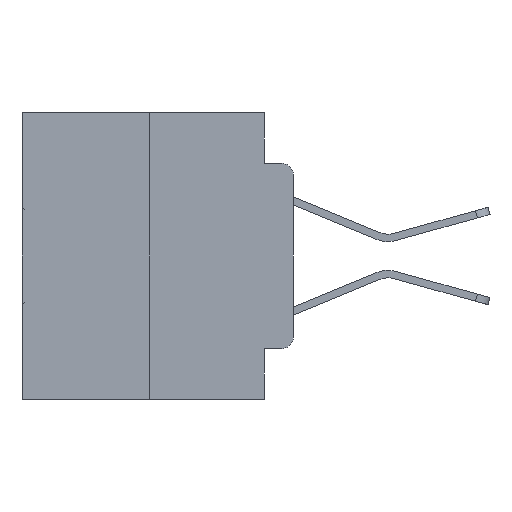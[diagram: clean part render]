
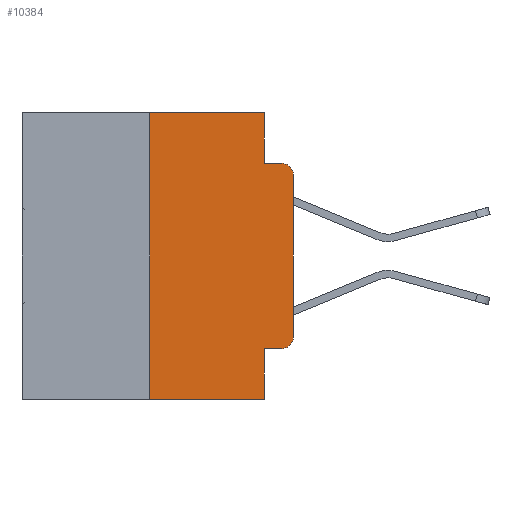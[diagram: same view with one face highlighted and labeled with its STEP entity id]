
A CAD part, left-side view. The second image highlights one B-rep face of the part: STEP entity #10384.
In plain terms, the highlighted planar face has unit normal (-1, 0, 0).
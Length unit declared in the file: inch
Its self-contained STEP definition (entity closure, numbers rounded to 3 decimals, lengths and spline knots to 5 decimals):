
#107 = EDGE_CURVE ( 'NONE', #1289, #26531, #20140, .T. ) ;
#1289 = VERTEX_POINT ( 'NONE', #2330 ) ;
#1302 = ORIENTED_EDGE ( 'NONE', *, *, #1705, .T. ) ;
#1594 = VERTEX_POINT ( 'NONE', #24197 ) ;
#1705 = EDGE_CURVE ( 'NONE', #2096, #1289, #15772, .T. ) ;
#2096 = VERTEX_POINT ( 'NONE', #21944 ) ;
#2208 = VECTOR ( 'NONE', #5639, 39.37008 ) ;
#2330 = CARTESIAN_POINT ( 'NONE',  ( 0., 0., -0.1085 ) ) ;
#2468 = DIRECTION ( 'NONE',  ( -1., 0., 0. ) ) ;
#3218 = CARTESIAN_POINT ( 'NONE',  ( 0., 0.051, -0.0885 ) ) ;
#3229 = CARTESIAN_POINT ( 'NONE',  ( 0., 0.473, 0. ) ) ;
#3512 = CARTESIAN_POINT ( 'NONE',  ( 0., 0.051, 0. ) ) ;
#3895 = VERTEX_POINT ( 'NONE', #10852 ) ;
#4520 = DIRECTION ( 'NONE',  ( 0., 0., -1. ) ) ;
#4838 = CARTESIAN_POINT ( 'NONE',  ( 0., 0.02, -0.3915 ) ) ;
#4951 = DIRECTION ( 'NONE',  ( 0., 0., -1. ) ) ;
#5204 = AXIS2_PLACEMENT_3D ( 'NONE', #11231, #2468, #21345 ) ;
#5575 = DIRECTION ( 'NONE',  ( 0., -1., 0. ) ) ;
#5639 = DIRECTION ( 'NONE',  ( 0., 0., 1. ) ) ;
#7127 = DIRECTION ( 'NONE',  ( 0., 0., -1. ) ) ;
#8042 = CARTESIAN_POINT ( 'NONE',  ( 0., 0.051, 0. ) ) ;
#8962 = VECTOR ( 'NONE', #20623, 39.37008 ) ;
#9237 = CARTESIAN_POINT ( 'NONE',  ( 0., 0.473, -0.5 ) ) ;
#9590 = ORIENTED_EDGE ( 'NONE', *, *, #24407, .F. ) ;
#10204 = VECTOR ( 'NONE', #18689, 39.37008 ) ;
#10384 = ADVANCED_FACE ( 'NONE', ( #26499 ), #29202, .F. ) ;
#10636 = LINE ( 'NONE', #16198, #27909 ) ;
#10852 = CARTESIAN_POINT ( 'NONE',  ( 0., 0.051, -0.4115 ) ) ;
#11231 = CARTESIAN_POINT ( 'NONE',  ( 0., 0.02, -0.1085 ) ) ;
#11590 = VECTOR ( 'NONE', #5575, 39.37008 ) ;
#13424 = ORIENTED_EDGE ( 'NONE', *, *, #26613, .F. ) ;
#13589 = LINE ( 'NONE', #19167, #2208 ) ;
#13669 = VECTOR ( 'NONE', #23942, 39.37008 ) ;
#13705 = CARTESIAN_POINT ( 'NONE',  ( 0., 0.051, -0.5 ) ) ;
#14106 = EDGE_LOOP ( 'NONE', ( #1302, #25506, #13424, #26874, #9590, #16303, #15659, #22327, #23051, #28242 ) ) ;
#14877 = EDGE_CURVE ( 'NONE', #19178, #26926, #21010, .T. ) ;
#15181 = CARTESIAN_POINT ( 'NONE',  ( 0., 0.25, -0.5 ) ) ;
#15219 = CIRCLE ( 'NONE', #21791, 0.02 ) ;
#15659 = ORIENTED_EDGE ( 'NONE', *, *, #14877, .T. ) ;
#15772 = LINE ( 'NONE', #27638, #22526 ) ;
#16022 = EDGE_CURVE ( 'NONE', #28334, #2096, #15219, .T. ) ;
#16198 = CARTESIAN_POINT ( 'NONE',  ( 0., 0.051, 0. ) ) ;
#16303 = ORIENTED_EDGE ( 'NONE', *, *, #22118, .F. ) ;
#16518 = CARTESIAN_POINT ( 'NONE',  ( 0., 0.02, -0.0885 ) ) ;
#17072 = VERTEX_POINT ( 'NONE', #8042 ) ;
#17523 = EDGE_CURVE ( 'NONE', #3895, #28334, #22249, .T. ) ;
#18047 = DIRECTION ( 'NONE',  ( 1., 0., 0. ) ) ;
#18689 = DIRECTION ( 'NONE',  ( 0., -1., 0. ) ) ;
#19080 = EDGE_CURVE ( 'NONE', #3895, #26926, #25731, .T. ) ;
#19167 = CARTESIAN_POINT ( 'NONE',  ( 0., 0.25, 0. ) ) ;
#19178 = VERTEX_POINT ( 'NONE', #15181 ) ;
#19844 = VERTEX_POINT ( 'NONE', #28662 ) ;
#20140 = CIRCLE ( 'NONE', #5204, 0.02 ) ;
#20623 = DIRECTION ( 'NONE',  ( 0., -1., 0. ) ) ;
#20663 = DIRECTION ( 'NONE',  ( -1., 0., 0. ) ) ;
#21010 = LINE ( 'NONE', #9237, #8962 ) ;
#21345 = DIRECTION ( 'NONE',  ( 0., 0., -1. ) ) ;
#21791 = AXIS2_PLACEMENT_3D ( 'NONE', #4838, #20663, #7127 ) ;
#21882 = AXIS2_PLACEMENT_3D ( 'NONE', #27011, #18047, #4520 ) ;
#21944 = CARTESIAN_POINT ( 'NONE',  ( 0., 0., -0.3915 ) ) ;
#22118 = EDGE_CURVE ( 'NONE', #19178, #1594, #13589, .T. ) ;
#22249 = LINE ( 'NONE', #27609, #10204 ) ;
#22327 = ORIENTED_EDGE ( 'NONE', *, *, #19080, .F. ) ;
#22526 = VECTOR ( 'NONE', #23301, 39.37008 ) ;
#22958 = LINE ( 'NONE', #3218, #11590 ) ;
#23051 = ORIENTED_EDGE ( 'NONE', *, *, #17523, .T. ) ;
#23301 = DIRECTION ( 'NONE',  ( 0., 0., 1. ) ) ;
#23942 = DIRECTION ( 'NONE',  ( 0., 0., -1. ) ) ;
#24197 = CARTESIAN_POINT ( 'NONE',  ( 0., 0.25, 0. ) ) ;
#24407 = EDGE_CURVE ( 'NONE', #1594, #17072, #25231, .T. ) ;
#24507 = VECTOR ( 'NONE', #28110, 39.37008 ) ;
#25152 = EDGE_CURVE ( 'NONE', #17072, #19844, #10636, .T. ) ;
#25231 = LINE ( 'NONE', #3229, #24507 ) ;
#25506 = ORIENTED_EDGE ( 'NONE', *, *, #107, .T. ) ;
#25731 = LINE ( 'NONE', #3512, #13669 ) ;
#25860 = CARTESIAN_POINT ( 'NONE',  ( 0., 0.02, -0.4115 ) ) ;
#26499 = FACE_OUTER_BOUND ( 'NONE', #14106, .T. ) ;
#26531 = VERTEX_POINT ( 'NONE', #16518 ) ;
#26613 = EDGE_CURVE ( 'NONE', #19844, #26531, #22958, .T. ) ;
#26874 = ORIENTED_EDGE ( 'NONE', *, *, #25152, .F. ) ;
#26926 = VERTEX_POINT ( 'NONE', #13705 ) ;
#27011 = CARTESIAN_POINT ( 'NONE',  ( 0., 0.473, 0. ) ) ;
#27609 = CARTESIAN_POINT ( 'NONE',  ( 0., 0.051, -0.4115 ) ) ;
#27638 = CARTESIAN_POINT ( 'NONE',  ( 0., 0., 0. ) ) ;
#27909 = VECTOR ( 'NONE', #4951, 39.37008 ) ;
#28110 = DIRECTION ( 'NONE',  ( 0., -1., 0. ) ) ;
#28242 = ORIENTED_EDGE ( 'NONE', *, *, #16022, .T. ) ;
#28334 = VERTEX_POINT ( 'NONE', #25860 ) ;
#28662 = CARTESIAN_POINT ( 'NONE',  ( 0., 0.051, -0.0885 ) ) ;
#29202 = PLANE ( 'NONE',  #21882 ) ;
